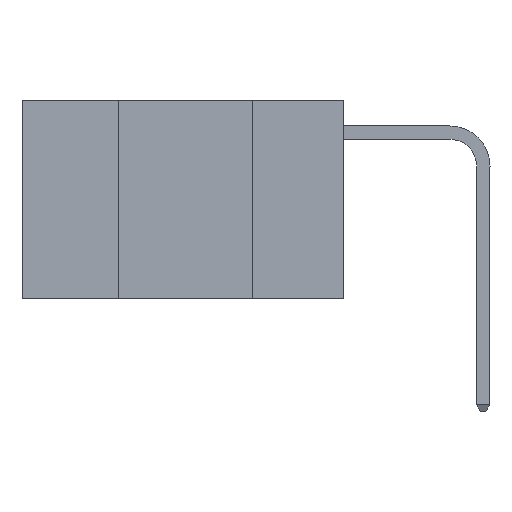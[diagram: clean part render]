
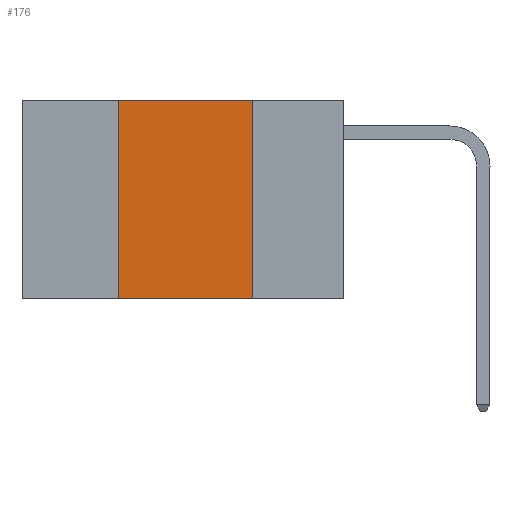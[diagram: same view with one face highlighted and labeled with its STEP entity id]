
A CAD part, left-side view. The second image highlights one B-rep face of the part: STEP entity #176.
In plain terms, the highlighted planar face has unit normal (-1, 0, 0).
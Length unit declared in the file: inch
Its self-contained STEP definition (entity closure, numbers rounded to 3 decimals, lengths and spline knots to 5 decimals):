
#176 = ADVANCED_FACE ( 'NONE', ( #4996 ), #2270, .F. ) ;
#679 = VERTEX_POINT ( 'NONE', #10471 ) ;
#838 = EDGE_CURVE ( 'NONE', #679, #5987, #8509, .T. ) ;
#895 = DIRECTION ( 'NONE',  ( 0., -1., 0. ) ) ;
#982 = CARTESIAN_POINT ( 'NONE',  ( 0., 0.6, 0. ) ) ;
#1860 = EDGE_CURVE ( 'NONE', #2208, #679, #3486, .T. ) ;
#2208 = VERTEX_POINT ( 'NONE', #10840 ) ;
#2270 = PLANE ( 'NONE',  #9224 ) ;
#3486 = LINE ( 'NONE', #982, #12915 ) ;
#4943 = ORIENTED_EDGE ( 'NONE', *, *, #11256, .T. ) ;
#4996 = FACE_OUTER_BOUND ( 'NONE', #11309, .T. ) ;
#5368 = VECTOR ( 'NONE', #12219, 39.37008 ) ;
#5615 = LINE ( 'NONE', #11230, #11165 ) ;
#5700 = LINE ( 'NONE', #8830, #8099 ) ;
#5987 = VERTEX_POINT ( 'NONE', #11842 ) ;
#6106 = VERTEX_POINT ( 'NONE', #13222 ) ;
#6960 = DIRECTION ( 'NONE',  ( 1., 0., 0. ) ) ;
#8099 = VECTOR ( 'NONE', #10014, 39.37008 ) ;
#8509 = LINE ( 'NONE', #12118, #5368 ) ;
#8830 = CARTESIAN_POINT ( 'NONE',  ( 0., 0.42, 0. ) ) ;
#9224 = AXIS2_PLACEMENT_3D ( 'NONE', #9350, #6960, #14035 ) ;
#9350 = CARTESIAN_POINT ( 'NONE',  ( 0., 0.6, 0. ) ) ;
#10014 = DIRECTION ( 'NONE',  ( 0., 0., 1. ) ) ;
#10471 = CARTESIAN_POINT ( 'NONE',  ( 0., 0.17, 0. ) ) ;
#10473 = ORIENTED_EDGE ( 'NONE', *, *, #838, .F. ) ;
#10721 = ORIENTED_EDGE ( 'NONE', *, *, #1860, .F. ) ;
#10840 = CARTESIAN_POINT ( 'NONE',  ( 0., 0.42, 0. ) ) ;
#11140 = ORIENTED_EDGE ( 'NONE', *, *, #14886, .F. ) ;
#11165 = VECTOR ( 'NONE', #12415, 39.37008 ) ;
#11230 = CARTESIAN_POINT ( 'NONE',  ( 0., 0.6, -0.37 ) ) ;
#11256 = EDGE_CURVE ( 'NONE', #6106, #5987, #5615, .T. ) ;
#11309 = EDGE_LOOP ( 'NONE', ( #10473, #10721, #11140, #4943 ) ) ;
#11842 = CARTESIAN_POINT ( 'NONE',  ( 0., 0.17, -0.37 ) ) ;
#12118 = CARTESIAN_POINT ( 'NONE',  ( 0., 0.17, 0. ) ) ;
#12219 = DIRECTION ( 'NONE',  ( 0., 0., -1. ) ) ;
#12415 = DIRECTION ( 'NONE',  ( 0., -1., 0. ) ) ;
#12915 = VECTOR ( 'NONE', #895, 39.37008 ) ;
#13222 = CARTESIAN_POINT ( 'NONE',  ( 0., 0.42, -0.37 ) ) ;
#14035 = DIRECTION ( 'NONE',  ( 0., 0., -1. ) ) ;
#14886 = EDGE_CURVE ( 'NONE', #6106, #2208, #5700, .T. ) ;
